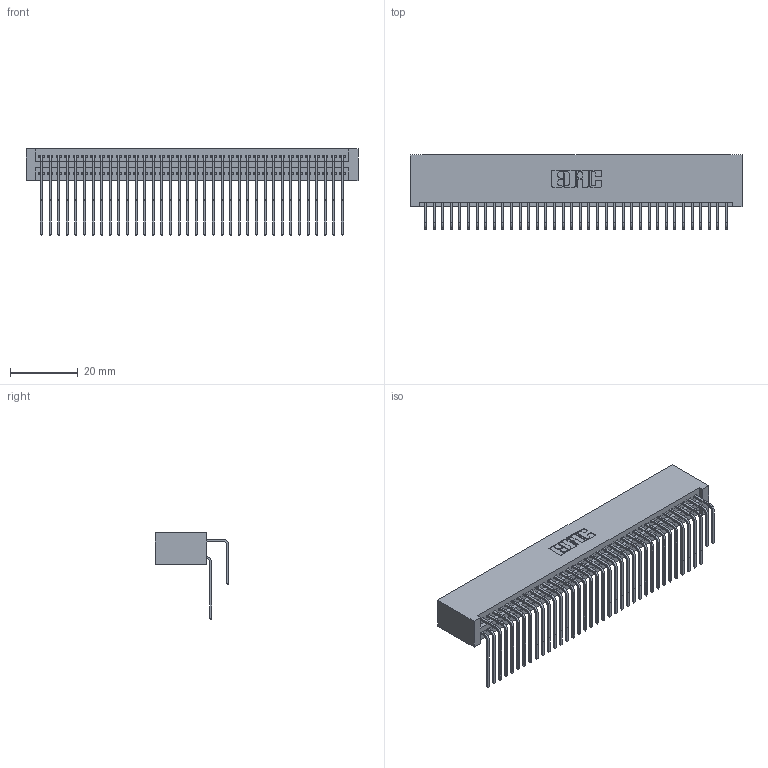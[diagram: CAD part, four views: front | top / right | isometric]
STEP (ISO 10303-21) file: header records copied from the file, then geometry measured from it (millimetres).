
FILE_DESCRIPTION (( 'STEP AP203' ), '1' );
FILE_NAME ('345-072-558-201.STEP', '2018-10-02T09:00:30', ( '' ), ( '' ), 'SwSTEP 2.0', 'SolidWorks 2016', '' );
FILE_SCHEMA (( 'CONFIG_CONTROL_DESIGN' ));
Length unit declared in the file: inch
Products named in the file (4): 345-292-001_558 559 Tail - 1; 345 Part_No Mounting Lugs; 345-292-001_558 Tail - 2; 345-072-558-201
Assembly tree (73 placements, depth 2):
  345-072-558-201
    345 Part_No Mounting Lugs
    345-292-001_558 559 Tail - 1  x36
    345-292-001_558 Tail - 2  x36
Bounding box: 98.04 x 21.83 x 25.53 mm (x, y, z)
Volume: 10499.7 mm3; surface area: 17660.4 mm2
Topology: 73 solids, 73 shells, 3862 faces, 11477 edges, 7554 vertices
Faces by surface type: plane 2596, cylinder 1266
Entity records: 30429 total; most frequent: CARTESIAN_POINT 5151, ORIENTED_EDGE 5034, DIRECTION 4517, EDGE_CURVE 2517, VECTOR 2209, LINE 2209, VERTEX_POINT 1674, AXIS2_PLACEMENT_3D 1154
